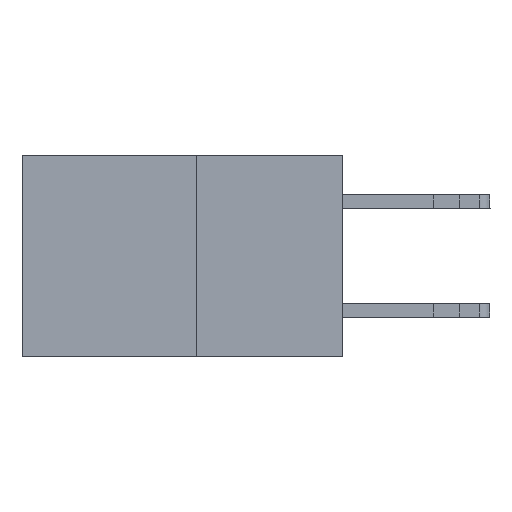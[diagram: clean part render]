
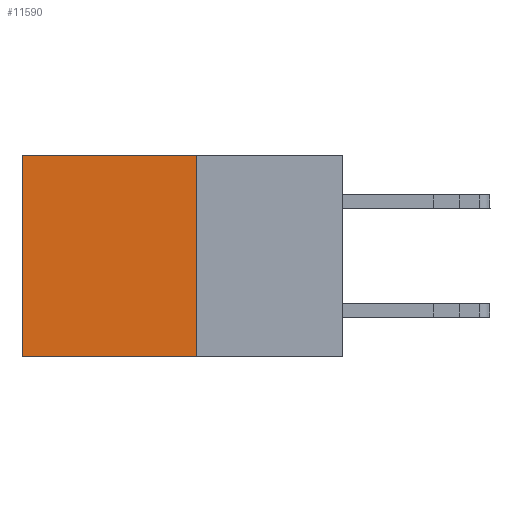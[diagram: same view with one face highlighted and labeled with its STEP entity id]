
A CAD part, left-side view. The second image highlights one B-rep face of the part: STEP entity #11590.
In plain terms, the highlighted planar face has unit normal (-1, 0, 0).
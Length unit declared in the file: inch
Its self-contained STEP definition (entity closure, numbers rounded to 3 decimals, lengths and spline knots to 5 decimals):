
#355 = EDGE_CURVE ( 'NONE', #1365, #14596, #18554, .T. ) ;
#1279 = CARTESIAN_POINT ( 'NONE',  ( 0.277, 0.27, 0. ) ) ;
#1365 = VERTEX_POINT ( 'NONE', #1279 ) ;
#2537 = CARTESIAN_POINT ( 'NONE',  ( 0.277, 0.27, 0. ) ) ;
#2753 = PLANE ( 'NONE',  #16560 ) ;
#3339 = EDGE_LOOP ( 'NONE', ( #11360, #17946, #14306, #13625 ) ) ;
#3428 = VECTOR ( 'NONE', #16548, 39.37008 ) ;
#3539 = LINE ( 'NONE', #12550, #18246 ) ;
#3920 = DIRECTION ( 'NONE',  ( 0., 1., 0. ) ) ;
#4223 = DIRECTION ( 'NONE',  ( 0., 0., -1. ) ) ;
#4800 = VECTOR ( 'NONE', #14423, 39.37008 ) ;
#5805 = CARTESIAN_POINT ( 'NONE',  ( 0.277, 0.59, -0.37 ) ) ;
#6236 = EDGE_CURVE ( 'NONE', #14596, #8977, #10234, .T. ) ;
#6876 = VECTOR ( 'NONE', #9841, 39.37008 ) ;
#8400 = CARTESIAN_POINT ( 'NONE',  ( 0.277, 0.59, -0.37 ) ) ;
#8977 = VERTEX_POINT ( 'NONE', #5805 ) ;
#9269 = VERTEX_POINT ( 'NONE', #12107 ) ;
#9841 = DIRECTION ( 'NONE',  ( 0., 0., -1. ) ) ;
#10234 = LINE ( 'NONE', #8400, #6876 ) ;
#11360 = ORIENTED_EDGE ( 'NONE', *, *, #6236, .T. ) ;
#11590 = ADVANCED_FACE ( 'NONE', ( #18340 ), #2753, .F. ) ;
#11709 = EDGE_CURVE ( 'NONE', #1365, #9269, #16240, .T. ) ;
#12107 = CARTESIAN_POINT ( 'NONE',  ( 0.277, 0.27, -0.37 ) ) ;
#12550 = CARTESIAN_POINT ( 'NONE',  ( 0.277, 0.27, -0.37 ) ) ;
#12830 = DIRECTION ( 'NONE',  ( 1., 0., 0. ) ) ;
#13014 = CARTESIAN_POINT ( 'NONE',  ( 0.277, 0.27, -0.37 ) ) ;
#13625 = ORIENTED_EDGE ( 'NONE', *, *, #355, .T. ) ;
#14306 = ORIENTED_EDGE ( 'NONE', *, *, #11709, .F. ) ;
#14423 = DIRECTION ( 'NONE',  ( 0., 0., -1. ) ) ;
#14596 = VERTEX_POINT ( 'NONE', #15020 ) ;
#15020 = CARTESIAN_POINT ( 'NONE',  ( 0.277, 0.59, 0. ) ) ;
#15652 = CARTESIAN_POINT ( 'NONE',  ( 0.277, 0.27, -0.37 ) ) ;
#16240 = LINE ( 'NONE', #13014, #4800 ) ;
#16355 = EDGE_CURVE ( 'NONE', #9269, #8977, #3539, .T. ) ;
#16548 = DIRECTION ( 'NONE',  ( 0., 1., 0. ) ) ;
#16560 = AXIS2_PLACEMENT_3D ( 'NONE', #15652, #12830, #4223 ) ;
#17946 = ORIENTED_EDGE ( 'NONE', *, *, #16355, .F. ) ;
#18246 = VECTOR ( 'NONE', #3920, 39.37008 ) ;
#18340 = FACE_OUTER_BOUND ( 'NONE', #3339, .T. ) ;
#18554 = LINE ( 'NONE', #2537, #3428 ) ;
